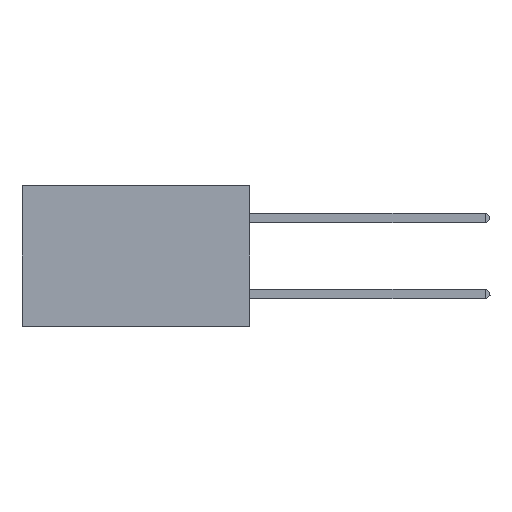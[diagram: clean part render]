
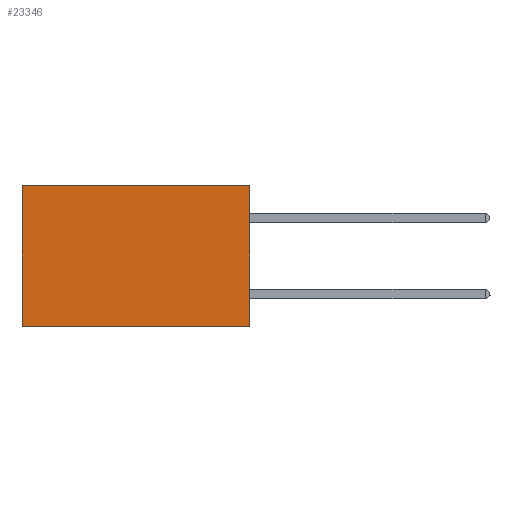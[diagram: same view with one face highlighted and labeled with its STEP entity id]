
A CAD part, left-side view. The second image highlights one B-rep face of the part: STEP entity #23346.
In plain terms, the highlighted planar face has unit normal (-1, 0, 0).
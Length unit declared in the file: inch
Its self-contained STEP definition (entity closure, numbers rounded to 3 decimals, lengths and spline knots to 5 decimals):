
#411 = CARTESIAN_POINT ( 'NONE',  ( 0.2875, 0.6, 0. ) ) ;
#617 = LINE ( 'NONE', #20564, #4908 ) ;
#1756 = CARTESIAN_POINT ( 'NONE',  ( 0.2875, 0.6, -0.37 ) ) ;
#1998 = LINE ( 'NONE', #2482, #25270 ) ;
#2482 = CARTESIAN_POINT ( 'NONE',  ( 0.2875, 0., -0.37 ) ) ;
#2551 = ORIENTED_EDGE ( 'NONE', *, *, #10969, .F. ) ;
#3874 = EDGE_CURVE ( 'NONE', #19132, #14004, #617, .T. ) ;
#4208 = CARTESIAN_POINT ( 'NONE',  ( 0.2875, 0.6, 0. ) ) ;
#4391 = DIRECTION ( 'NONE',  ( 0., 0., -1. ) ) ;
#4908 = VECTOR ( 'NONE', #6630, 39.37008 ) ;
#5529 = ORIENTED_EDGE ( 'NONE', *, *, #8049, .T. ) ;
#6511 = CARTESIAN_POINT ( 'NONE',  ( 0.2875, 0., 0. ) ) ;
#6630 = DIRECTION ( 'NONE',  ( 0., 1., 0. ) ) ;
#7322 = LINE ( 'NONE', #25190, #13136 ) ;
#8049 = EDGE_CURVE ( 'NONE', #14004, #8778, #11261, .T. ) ;
#8457 = CARTESIAN_POINT ( 'NONE',  ( 0.2875, 0., -0.37 ) ) ;
#8661 = ORIENTED_EDGE ( 'NONE', *, *, #23442, .F. ) ;
#8778 = VERTEX_POINT ( 'NONE', #1756 ) ;
#8868 = EDGE_LOOP ( 'NONE', ( #5529, #2551, #8661, #22196 ) ) ;
#10969 = EDGE_CURVE ( 'NONE', #17740, #8778, #1998, .T. ) ;
#11261 = LINE ( 'NONE', #411, #24419 ) ;
#13136 = VECTOR ( 'NONE', #23040, 39.37008 ) ;
#13996 = DIRECTION ( 'NONE',  ( 0., 0., -1. ) ) ;
#14004 = VERTEX_POINT ( 'NONE', #4208 ) ;
#17740 = VERTEX_POINT ( 'NONE', #8457 ) ;
#19132 = VERTEX_POINT ( 'NONE', #6511 ) ;
#20480 = CARTESIAN_POINT ( 'NONE',  ( 0.2875, 0., 0. ) ) ;
#20564 = CARTESIAN_POINT ( 'NONE',  ( 0.2875, 0., 0. ) ) ;
#20870 = DIRECTION ( 'NONE',  ( 1., 0., 0. ) ) ;
#22196 = ORIENTED_EDGE ( 'NONE', *, *, #3874, .T. ) ;
#23040 = DIRECTION ( 'NONE',  ( 0., 0., -1. ) ) ;
#23346 = ADVANCED_FACE ( 'NONE', ( #25209 ), #27911, .F. ) ;
#23442 = EDGE_CURVE ( 'NONE', #19132, #17740, #7322, .T. ) ;
#24276 = AXIS2_PLACEMENT_3D ( 'NONE', #20480, #20870, #4391 ) ;
#24419 = VECTOR ( 'NONE', #13996, 39.37008 ) ;
#25190 = CARTESIAN_POINT ( 'NONE',  ( 0.2875, 0., 0. ) ) ;
#25209 = FACE_OUTER_BOUND ( 'NONE', #8868, .T. ) ;
#25270 = VECTOR ( 'NONE', #25756, 39.37008 ) ;
#25756 = DIRECTION ( 'NONE',  ( 0., 1., 0. ) ) ;
#27911 = PLANE ( 'NONE',  #24276 ) ;
